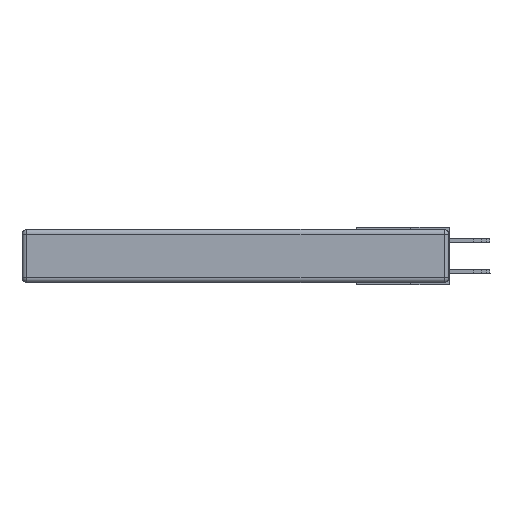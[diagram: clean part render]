
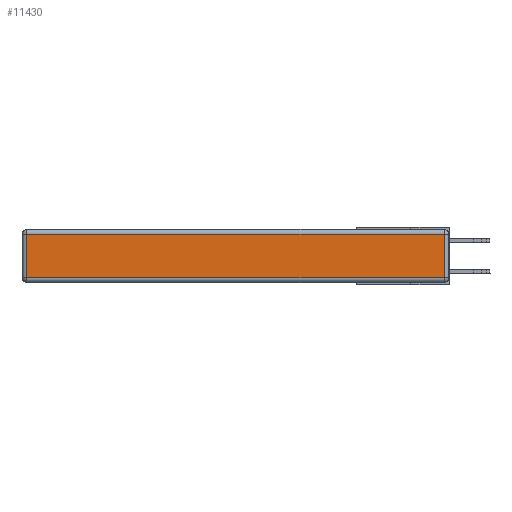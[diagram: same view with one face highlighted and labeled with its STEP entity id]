
A CAD part, left-side view. The second image highlights one B-rep face of the part: STEP entity #11430.
In plain terms, the highlighted planar face has unit normal (-1, 0, 0).
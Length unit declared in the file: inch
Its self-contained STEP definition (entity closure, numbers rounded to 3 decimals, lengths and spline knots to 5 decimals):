
#153 = CARTESIAN_POINT ( 'NONE',  ( 0., 2.72, -0.313 ) ) ;
#157 = LINE ( 'NONE', #4660, #13360 ) ;
#251 = CARTESIAN_POINT ( 'NONE',  ( 0., 0.03, -0.313 ) ) ;
#817 = DIRECTION ( 'NONE',  ( 0., 0., -1. ) ) ;
#978 = CARTESIAN_POINT ( 'NONE',  ( 0., 0.03, -0.03 ) ) ;
#2550 = AXIS2_PLACEMENT_3D ( 'NONE', #4456, #11761, #15850 ) ;
#4456 = CARTESIAN_POINT ( 'NONE',  ( 0., 0., -0.343 ) ) ;
#4660 = CARTESIAN_POINT ( 'NONE',  ( 0., 2.72, -0.343 ) ) ;
#5846 = EDGE_CURVE ( 'NONE', #18996, #13558, #7210, .T. ) ;
#6725 = ORIENTED_EDGE ( 'NONE', *, *, #15586, .T. ) ;
#6939 = FACE_OUTER_BOUND ( 'NONE', #20244, .T. ) ;
#7210 = LINE ( 'NONE', #9412, #13384 ) ;
#7940 = VECTOR ( 'NONE', #21049, 39.37008 ) ;
#7999 = ORIENTED_EDGE ( 'NONE', *, *, #5846, .T. ) ;
#8820 = VERTEX_POINT ( 'NONE', #978 ) ;
#9048 = LINE ( 'NONE', #16581, #11967 ) ;
#9412 = CARTESIAN_POINT ( 'NONE',  ( 0., 0., -0.313 ) ) ;
#11430 = ADVANCED_FACE ( 'NONE', ( #6939 ), #17624, .T. ) ;
#11731 = LINE ( 'NONE', #21198, #7940 ) ;
#11761 = DIRECTION ( 'NONE',  ( -1., 0., 0. ) ) ;
#11967 = VECTOR ( 'NONE', #18907, 39.37008 ) ;
#13360 = VECTOR ( 'NONE', #817, 39.37008 ) ;
#13384 = VECTOR ( 'NONE', #22417, 39.37008 ) ;
#13558 = VERTEX_POINT ( 'NONE', #251 ) ;
#13675 = VERTEX_POINT ( 'NONE', #23635 ) ;
#14246 = ORIENTED_EDGE ( 'NONE', *, *, #18636, .T. ) ;
#15586 = EDGE_CURVE ( 'NONE', #13675, #18996, #157, .T. ) ;
#15850 = DIRECTION ( 'NONE',  ( 0., 0., 1. ) ) ;
#16581 = CARTESIAN_POINT ( 'NONE',  ( 0., 2.75, -0.03 ) ) ;
#17624 = PLANE ( 'NONE',  #2550 ) ;
#18636 = EDGE_CURVE ( 'NONE', #13558, #8820, #11731, .T. ) ;
#18907 = DIRECTION ( 'NONE',  ( 0., 1., 0. ) ) ;
#18996 = VERTEX_POINT ( 'NONE', #153 ) ;
#19912 = EDGE_CURVE ( 'NONE', #8820, #13675, #9048, .T. ) ;
#20244 = EDGE_LOOP ( 'NONE', ( #7999, #14246, #23218, #6725 ) ) ;
#21049 = DIRECTION ( 'NONE',  ( 0., 0., 1. ) ) ;
#21198 = CARTESIAN_POINT ( 'NONE',  ( 0., 0.03, -0.343 ) ) ;
#22417 = DIRECTION ( 'NONE',  ( 0., -1., 0. ) ) ;
#23218 = ORIENTED_EDGE ( 'NONE', *, *, #19912, .T. ) ;
#23635 = CARTESIAN_POINT ( 'NONE',  ( 0., 2.72, -0.03 ) ) ;
